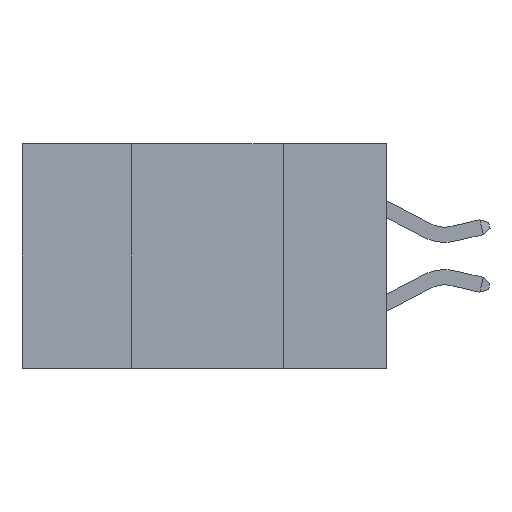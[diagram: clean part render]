
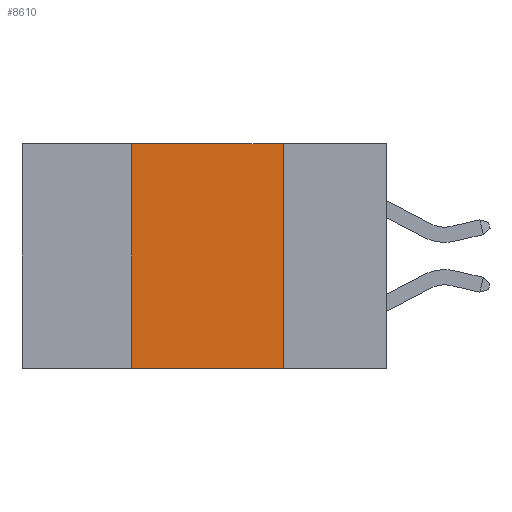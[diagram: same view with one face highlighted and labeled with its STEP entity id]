
A CAD part, left-side view. The second image highlights one B-rep face of the part: STEP entity #8610.
In plain terms, the highlighted planar face has unit normal (-1, 0, 0).
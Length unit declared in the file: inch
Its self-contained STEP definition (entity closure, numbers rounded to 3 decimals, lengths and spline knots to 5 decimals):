
#777 = ORIENTED_EDGE ( 'NONE', *, *, #9623, .F. ) ;
#782 = DIRECTION ( 'NONE',  ( 0., 0., -1. ) ) ;
#1055 = CARTESIAN_POINT ( 'NONE',  ( 0., 0.42, 0. ) ) ;
#1127 = ORIENTED_EDGE ( 'NONE', *, *, #10713, .T. ) ;
#1505 = VERTEX_POINT ( 'NONE', #11454 ) ;
#1697 = VERTEX_POINT ( 'NONE', #6300 ) ;
#1708 = CARTESIAN_POINT ( 'NONE',  ( 0., 0.6, 0. ) ) ;
#2101 = EDGE_LOOP ( 'NONE', ( #4525, #9197, #777, #1127 ) ) ;
#2312 = DIRECTION ( 'NONE',  ( 0., 0., -1. ) ) ;
#2574 = CARTESIAN_POINT ( 'NONE',  ( 0., 0.17, -0.37 ) ) ;
#2631 = DIRECTION ( 'NONE',  ( 0., -1., 0. ) ) ;
#4525 = ORIENTED_EDGE ( 'NONE', *, *, #9055, .F. ) ;
#5113 = PLANE ( 'NONE',  #8695 ) ;
#5221 = LINE ( 'NONE', #1055, #10144 ) ;
#6300 = CARTESIAN_POINT ( 'NONE',  ( 0., 0.42, 0. ) ) ;
#6460 = CARTESIAN_POINT ( 'NONE',  ( 0., 0.6, -0.37 ) ) ;
#6670 = FACE_OUTER_BOUND ( 'NONE', #2101, .T. ) ;
#7578 = DIRECTION ( 'NONE',  ( 0., 0., 1. ) ) ;
#7823 = DIRECTION ( 'NONE',  ( 1., 0., 0. ) ) ;
#7992 = VECTOR ( 'NONE', #8202, 39.37008 ) ;
#8166 = VECTOR ( 'NONE', #782, 39.37008 ) ;
#8202 = DIRECTION ( 'NONE',  ( 0., -1., 0. ) ) ;
#8259 = CARTESIAN_POINT ( 'NONE',  ( 0., 0.17, 0. ) ) ;
#8279 = VECTOR ( 'NONE', #2631, 39.37008 ) ;
#8610 = ADVANCED_FACE ( 'NONE', ( #6670 ), #5113, .F. ) ;
#8695 = AXIS2_PLACEMENT_3D ( 'NONE', #11129, #7823, #2312 ) ;
#8786 = CARTESIAN_POINT ( 'NONE',  ( 0., 0.17, 0. ) ) ;
#9055 = EDGE_CURVE ( 'NONE', #9792, #9345, #10651, .T. ) ;
#9197 = ORIENTED_EDGE ( 'NONE', *, *, #10655, .F. ) ;
#9345 = VERTEX_POINT ( 'NONE', #2574 ) ;
#9623 = EDGE_CURVE ( 'NONE', #1505, #1697, #5221, .T. ) ;
#9792 = VERTEX_POINT ( 'NONE', #8786 ) ;
#10144 = VECTOR ( 'NONE', #7578, 39.37008 ) ;
#10501 = LINE ( 'NONE', #1708, #8279 ) ;
#10651 = LINE ( 'NONE', #8259, #8166 ) ;
#10655 = EDGE_CURVE ( 'NONE', #1697, #9792, #10501, .T. ) ;
#10713 = EDGE_CURVE ( 'NONE', #1505, #9345, #10980, .T. ) ;
#10980 = LINE ( 'NONE', #6460, #7992 ) ;
#11129 = CARTESIAN_POINT ( 'NONE',  ( 0., 0.6, 0. ) ) ;
#11454 = CARTESIAN_POINT ( 'NONE',  ( 0., 0.42, -0.37 ) ) ;
